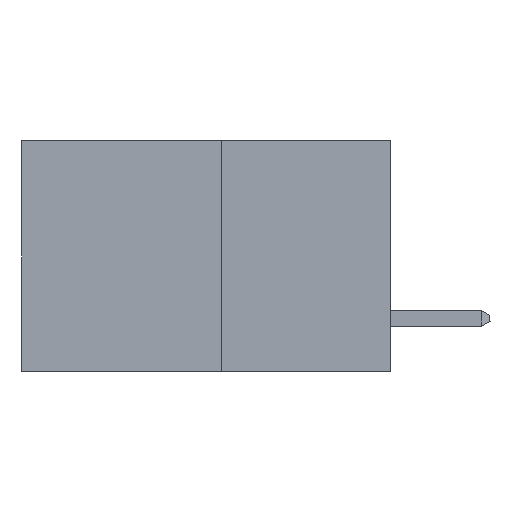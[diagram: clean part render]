
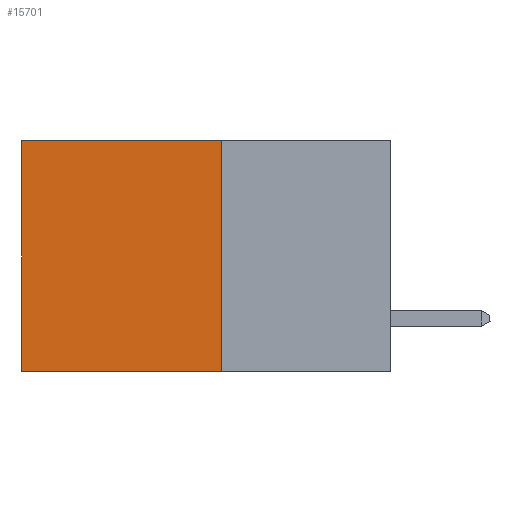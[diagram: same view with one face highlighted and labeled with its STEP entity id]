
A CAD part, left-side view. The second image highlights one B-rep face of the part: STEP entity #15701.
In plain terms, the highlighted planar face has unit normal (-1, 0, 0).
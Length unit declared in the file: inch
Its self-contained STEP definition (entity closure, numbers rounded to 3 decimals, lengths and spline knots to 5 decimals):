
#331 = VERTEX_POINT ( 'NONE', #1951 ) ;
#458 = DIRECTION ( 'NONE',  ( 0., 1., 0. ) ) ;
#1102 = CARTESIAN_POINT ( 'NONE',  ( 0.277, 0.27, 0. ) ) ;
#1217 = PLANE ( 'NONE',  #9673 ) ;
#1319 = VECTOR ( 'NONE', #6674, 39.37008 ) ;
#1951 = CARTESIAN_POINT ( 'NONE',  ( 0.277, 0.27, -0.37 ) ) ;
#2389 = ORIENTED_EDGE ( 'NONE', *, *, #14461, .T. ) ;
#2734 = DIRECTION ( 'NONE',  ( 1., 0., 0. ) ) ;
#2804 = CARTESIAN_POINT ( 'NONE',  ( 0.277, 0.27, 0. ) ) ;
#3541 = CARTESIAN_POINT ( 'NONE',  ( 0.277, 0.27, -0.37 ) ) ;
#4765 = LINE ( 'NONE', #8642, #15886 ) ;
#4801 = EDGE_CURVE ( 'NONE', #9143, #14680, #4765, .T. ) ;
#5410 = LINE ( 'NONE', #3541, #1319 ) ;
#5621 = DIRECTION ( 'NONE',  ( 0., 0., -1. ) ) ;
#5662 = VECTOR ( 'NONE', #458, 39.37008 ) ;
#6674 = DIRECTION ( 'NONE',  ( 0., 0., -1. ) ) ;
#6914 = EDGE_LOOP ( 'NONE', ( #7709, #11693, #8664, #2389 ) ) ;
#7177 = EDGE_CURVE ( 'NONE', #331, #14680, #13710, .T. ) ;
#7709 = ORIENTED_EDGE ( 'NONE', *, *, #4801, .T. ) ;
#7782 = CARTESIAN_POINT ( 'NONE',  ( 0.277, 0.59, -0.37 ) ) ;
#8112 = VERTEX_POINT ( 'NONE', #1102 ) ;
#8642 = CARTESIAN_POINT ( 'NONE',  ( 0.277, 0.59, -0.37 ) ) ;
#8664 = ORIENTED_EDGE ( 'NONE', *, *, #9496, .F. ) ;
#9143 = VERTEX_POINT ( 'NONE', #10382 ) ;
#9496 = EDGE_CURVE ( 'NONE', #8112, #331, #5410, .T. ) ;
#9673 = AXIS2_PLACEMENT_3D ( 'NONE', #11878, #2734, #13408 ) ;
#10382 = CARTESIAN_POINT ( 'NONE',  ( 0.277, 0.59, 0. ) ) ;
#10442 = DIRECTION ( 'NONE',  ( 0., 1., 0. ) ) ;
#10693 = FACE_OUTER_BOUND ( 'NONE', #6914, .T. ) ;
#11693 = ORIENTED_EDGE ( 'NONE', *, *, #7177, .F. ) ;
#11878 = CARTESIAN_POINT ( 'NONE',  ( 0.277, 0.27, -0.37 ) ) ;
#13408 = DIRECTION ( 'NONE',  ( 0., 0., -1. ) ) ;
#13710 = LINE ( 'NONE', #17083, #5662 ) ;
#14288 = LINE ( 'NONE', #2804, #14748 ) ;
#14461 = EDGE_CURVE ( 'NONE', #8112, #9143, #14288, .T. ) ;
#14680 = VERTEX_POINT ( 'NONE', #7782 ) ;
#14748 = VECTOR ( 'NONE', #10442, 39.37008 ) ;
#15701 = ADVANCED_FACE ( 'NONE', ( #10693 ), #1217, .F. ) ;
#15886 = VECTOR ( 'NONE', #5621, 39.37008 ) ;
#17083 = CARTESIAN_POINT ( 'NONE',  ( 0.277, 0.27, -0.37 ) ) ;
